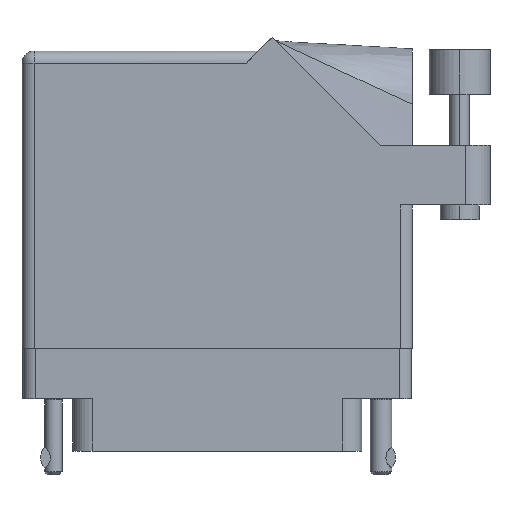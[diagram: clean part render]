
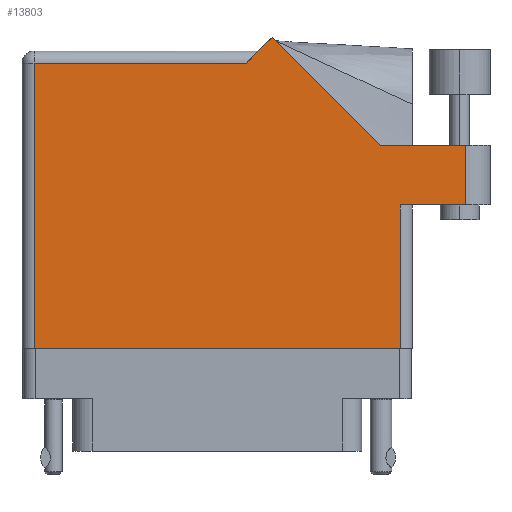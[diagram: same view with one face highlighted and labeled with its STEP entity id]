
A CAD part, front view. The second image highlights one B-rep face of the part: STEP entity #13803.
In plain terms, the highlighted face is planar.
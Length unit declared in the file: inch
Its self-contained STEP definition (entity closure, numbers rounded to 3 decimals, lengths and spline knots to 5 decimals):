
#858 = EDGE_LOOP ( 'NONE', ( #32871, #16886, #46599, #16449, #25502, #44430, #43004, #26102, #9676 ) ) ;
#2875 = CARTESIAN_POINT ( 'NONE',  ( 2.285, 0.737, 0. ) ) ;
#3027 = VECTOR ( 'NONE', #4451, 39.37008 ) ;
#3428 = PLANE ( 'NONE',  #18150 ) ;
#4451 = DIRECTION ( 'NONE',  ( 1., 0., 0. ) ) ;
#4846 = DIRECTION ( 'NONE',  ( 0., 1., 0. ) ) ;
#5526 = CARTESIAN_POINT ( 'NONE',  ( 1.84442, 1.044, 0. ) ) ;
#6103 = CARTESIAN_POINT ( 'NONE',  ( 2.285, 1.044, 0. ) ) ;
#6132 = VERTEX_POINT ( 'NONE', #32700 ) ;
#6164 = LINE ( 'NONE', #47222, #35809 ) ;
#6678 = VERTEX_POINT ( 'NONE', #6103 ) ;
#6717 = CARTESIAN_POINT ( 'NONE',  ( 0., 1.468, 0. ) ) ;
#7170 = DIRECTION ( 'NONE',  ( 0., 0., -1. ) ) ;
#7511 = EDGE_CURVE ( 'NONE', #44878, #6678, #31668, .T. ) ;
#7756 = CARTESIAN_POINT ( 'NONE',  ( 1.155, 1.468, 0. ) ) ;
#8088 = VERTEX_POINT ( 'NONE', #22776 ) ;
#8821 = CARTESIAN_POINT ( 'NONE',  ( 0., 0., 0. ) ) ;
#8996 = EDGE_CURVE ( 'NONE', #20869, #15814, #15246, .T. ) ;
#9658 = EDGE_CURVE ( 'NONE', #16633, #44878, #37346, .T. ) ;
#9664 = DIRECTION ( 'NONE',  ( 0., 1., 0. ) ) ;
#9676 = ORIENTED_EDGE ( 'NONE', *, *, #28800, .T. ) ;
#9919 = CARTESIAN_POINT ( 'NONE',  ( 1.948, 0.737, 0. ) ) ;
#10540 = LINE ( 'NONE', #10655, #47765 ) ;
#10655 = CARTESIAN_POINT ( 'NONE',  ( 0.062, 0., 0. ) ) ;
#11989 = VERTEX_POINT ( 'NONE', #44216 ) ;
#12847 = VECTOR ( 'NONE', #29186, 39.37008 ) ;
#13729 = CARTESIAN_POINT ( 'NONE',  ( 1.948, 0., 0. ) ) ;
#13803 = ADVANCED_FACE ( 'NONE', ( #15647 ), #3428, .F. ) ;
#14692 = DIRECTION ( 'NONE',  ( 0., -1., 0. ) ) ;
#15246 = LINE ( 'NONE', #27450, #39122 ) ;
#15535 = CARTESIAN_POINT ( 'NONE',  ( 2.285, 1.044, 0. ) ) ;
#15647 = FACE_OUTER_BOUND ( 'NONE', #858, .T. ) ;
#15814 = VERTEX_POINT ( 'NONE', #7756 ) ;
#15947 = VECTOR ( 'NONE', #40068, 39.37008 ) ;
#16449 = ORIENTED_EDGE ( 'NONE', *, *, #26225, .T. ) ;
#16633 = VERTEX_POINT ( 'NONE', #9919 ) ;
#16886 = ORIENTED_EDGE ( 'NONE', *, *, #7511, .T. ) ;
#18150 = AXIS2_PLACEMENT_3D ( 'NONE', #29406, #7170, #21888 ) ;
#20869 = VERTEX_POINT ( 'NONE', #21934 ) ;
#21888 = DIRECTION ( 'NONE',  ( -1., 0., 0. ) ) ;
#21934 = CARTESIAN_POINT ( 'NONE',  ( 1.28771, 1.60071, 0. ) ) ;
#22739 = LINE ( 'NONE', #8821, #3027 ) ;
#22776 = CARTESIAN_POINT ( 'NONE',  ( 1.84442, 1.044, 0. ) ) ;
#24531 = EDGE_CURVE ( 'NONE', #15814, #6132, #41041, .T. ) ;
#25502 = ORIENTED_EDGE ( 'NONE', *, *, #8996, .T. ) ;
#26102 = ORIENTED_EDGE ( 'NONE', *, *, #32906, .T. ) ;
#26225 = EDGE_CURVE ( 'NONE', #8088, #20869, #46665, .T. ) ;
#26363 = EDGE_CURVE ( 'NONE', #6678, #8088, #32444, .T. ) ;
#26974 = VECTOR ( 'NONE', #4846, 39.37008 ) ;
#27450 = CARTESIAN_POINT ( 'NONE',  ( 1.217, 1.53, 0. ) ) ;
#28061 = DIRECTION ( 'NONE',  ( -0.707, 0.707, 0. ) ) ;
#28800 = EDGE_CURVE ( 'NONE', #42649, #16633, #6164, .T. ) ;
#29186 = DIRECTION ( 'NONE',  ( 1., 0., 0. ) ) ;
#29406 = CARTESIAN_POINT ( 'NONE',  ( 0., 1.53, 0. ) ) ;
#31668 = LINE ( 'NONE', #15535, #26974 ) ;
#32311 = CARTESIAN_POINT ( 'NONE',  ( 2.41, 1.044, 0. ) ) ;
#32444 = LINE ( 'NONE', #32311, #40534 ) ;
#32464 = DIRECTION ( 'NONE',  ( -1., 0., 0. ) ) ;
#32700 = CARTESIAN_POINT ( 'NONE',  ( 0.062, 1.468, 0. ) ) ;
#32871 = ORIENTED_EDGE ( 'NONE', *, *, #9658, .T. ) ;
#32906 = EDGE_CURVE ( 'NONE', #11989, #42649, #22739, .T. ) ;
#35809 = VECTOR ( 'NONE', #9664, 39.37008 ) ;
#36792 = VECTOR ( 'NONE', #28061, 39.37008 ) ;
#37346 = LINE ( 'NONE', #40295, #12847 ) ;
#39122 = VECTOR ( 'NONE', #45849, 39.37008 ) ;
#40068 = DIRECTION ( 'NONE',  ( -1., 0., 0. ) ) ;
#40295 = CARTESIAN_POINT ( 'NONE',  ( 2.01, 0.737, 0. ) ) ;
#40534 = VECTOR ( 'NONE', #32464, 39.37008 ) ;
#41041 = LINE ( 'NONE', #6717, #15947 ) ;
#42649 = VERTEX_POINT ( 'NONE', #13729 ) ;
#43004 = ORIENTED_EDGE ( 'NONE', *, *, #43933, .T. ) ;
#43933 = EDGE_CURVE ( 'NONE', #6132, #11989, #10540, .T. ) ;
#44216 = CARTESIAN_POINT ( 'NONE',  ( 0.062, 0., 0. ) ) ;
#44430 = ORIENTED_EDGE ( 'NONE', *, *, #24531, .T. ) ;
#44878 = VERTEX_POINT ( 'NONE', #2875 ) ;
#45849 = DIRECTION ( 'NONE',  ( -0.707, -0.707, 0. ) ) ;
#46599 = ORIENTED_EDGE ( 'NONE', *, *, #26363, .T. ) ;
#46665 = LINE ( 'NONE', #5526, #36792 ) ;
#47222 = CARTESIAN_POINT ( 'NONE',  ( 1.948, 0.737, 0. ) ) ;
#47765 = VECTOR ( 'NONE', #14692, 39.37008 ) ;
